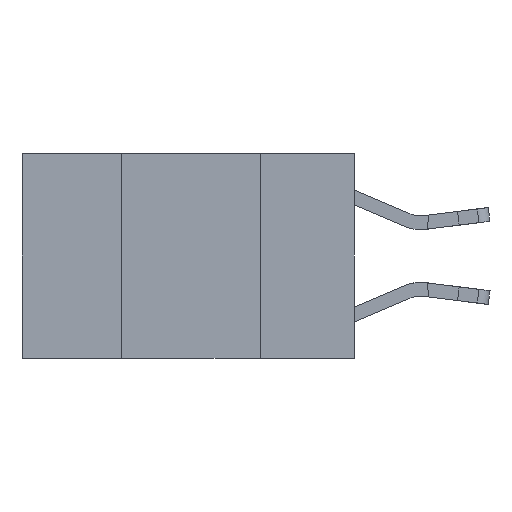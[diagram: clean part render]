
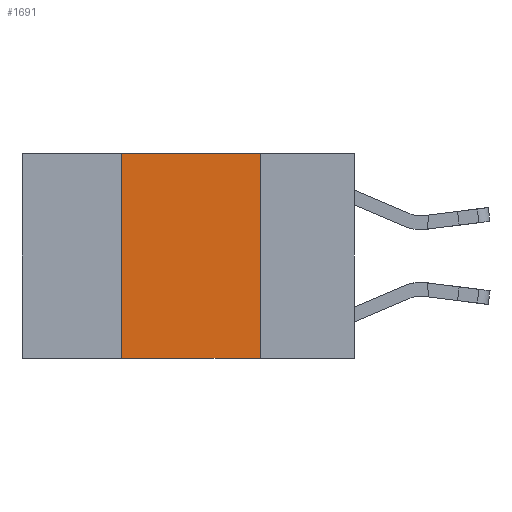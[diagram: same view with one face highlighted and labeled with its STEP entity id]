
A CAD part, left-side view. The second image highlights one B-rep face of the part: STEP entity #1691.
In plain terms, the highlighted planar face has unit normal (-1, 0, 0).
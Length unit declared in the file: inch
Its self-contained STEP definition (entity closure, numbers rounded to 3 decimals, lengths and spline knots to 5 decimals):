
#454 = AXIS2_PLACEMENT_3D ( 'NONE', #2670, #9641, #11038 ) ;
#462 = FACE_OUTER_BOUND ( 'NONE', #10292, .T. ) ;
#742 = LINE ( 'NONE', #3130, #9731 ) ;
#1114 = EDGE_CURVE ( 'NONE', #7167, #11096, #8962, .T. ) ;
#1691 = ADVANCED_FACE ( 'NONE', ( #462 ), #5058, .F. ) ;
#2053 = CARTESIAN_POINT ( 'NONE',  ( 0., 0.17, 0. ) ) ;
#2670 = CARTESIAN_POINT ( 'NONE',  ( 0., 0.6, 0. ) ) ;
#2852 = VERTEX_POINT ( 'NONE', #12734 ) ;
#3130 = CARTESIAN_POINT ( 'NONE',  ( 0., 0.6, -0.37 ) ) ;
#3264 = DIRECTION ( 'NONE',  ( 0., 0., -1. ) ) ;
#4093 = VECTOR ( 'NONE', #3264, 39.37008 ) ;
#4344 = CARTESIAN_POINT ( 'NONE',  ( 0., 0.42, 0. ) ) ;
#4772 = VECTOR ( 'NONE', #9043, 39.37008 ) ;
#5058 = PLANE ( 'NONE',  #454 ) ;
#5336 = EDGE_CURVE ( 'NONE', #11096, #2852, #10492, .T. ) ;
#5715 = ORIENTED_EDGE ( 'NONE', *, *, #12428, .F. ) ;
#6087 = VERTEX_POINT ( 'NONE', #11516 ) ;
#6125 = CARTESIAN_POINT ( 'NONE',  ( 0., 0.6, 0. ) ) ;
#6221 = DIRECTION ( 'NONE',  ( 0., -1., 0. ) ) ;
#7167 = VERTEX_POINT ( 'NONE', #4344 ) ;
#7876 = CARTESIAN_POINT ( 'NONE',  ( 0., 0.17, 0. ) ) ;
#7905 = CARTESIAN_POINT ( 'NONE',  ( 0., 0.42, 0. ) ) ;
#8716 = ORIENTED_EDGE ( 'NONE', *, *, #13124, .T. ) ;
#8890 = DIRECTION ( 'NONE',  ( 0., -1., 0. ) ) ;
#8962 = LINE ( 'NONE', #6125, #11926 ) ;
#9043 = DIRECTION ( 'NONE',  ( 0., 0., 1. ) ) ;
#9641 = DIRECTION ( 'NONE',  ( 1., 0., 0. ) ) ;
#9731 = VECTOR ( 'NONE', #8890, 39.37008 ) ;
#10292 = EDGE_LOOP ( 'NONE', ( #11834, #12183, #5715, #8716 ) ) ;
#10492 = LINE ( 'NONE', #2053, #4093 ) ;
#11038 = DIRECTION ( 'NONE',  ( 0., 0., -1. ) ) ;
#11096 = VERTEX_POINT ( 'NONE', #7876 ) ;
#11516 = CARTESIAN_POINT ( 'NONE',  ( 0., 0.42, -0.37 ) ) ;
#11834 = ORIENTED_EDGE ( 'NONE', *, *, #5336, .F. ) ;
#11926 = VECTOR ( 'NONE', #6221, 39.37008 ) ;
#12183 = ORIENTED_EDGE ( 'NONE', *, *, #1114, .F. ) ;
#12428 = EDGE_CURVE ( 'NONE', #6087, #7167, #13760, .T. ) ;
#12734 = CARTESIAN_POINT ( 'NONE',  ( 0., 0.17, -0.37 ) ) ;
#13124 = EDGE_CURVE ( 'NONE', #6087, #2852, #742, .T. ) ;
#13760 = LINE ( 'NONE', #7905, #4772 ) ;
